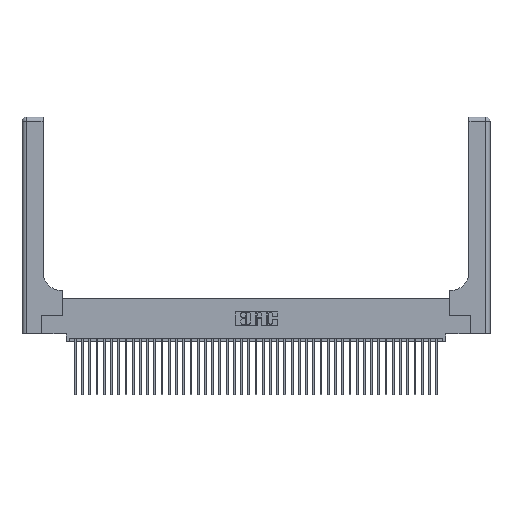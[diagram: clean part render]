
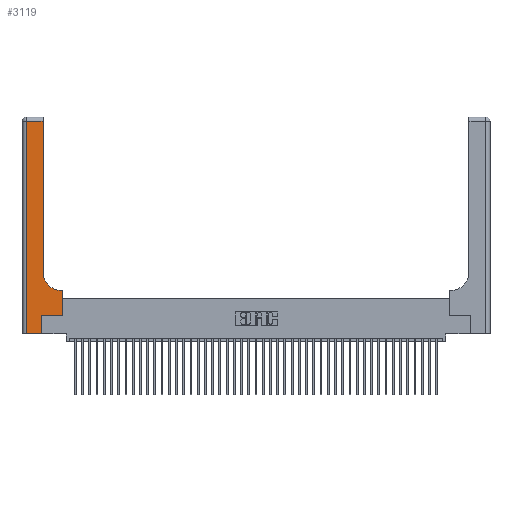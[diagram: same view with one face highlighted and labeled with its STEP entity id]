
A CAD part, top view. The second image highlights one B-rep face of the part: STEP entity #3119.
In plain terms, the highlighted planar face has unit normal (0, 0, 1).
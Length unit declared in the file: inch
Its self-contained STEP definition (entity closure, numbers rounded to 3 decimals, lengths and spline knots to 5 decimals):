
#1392 = CARTESIAN_POINT ( 'NONE',  ( 0.5415, 0.85, 0.37 ) ) ;
#1647 = DIRECTION ( 'NONE',  ( 0., 1., 0. ) ) ;
#1815 = CARTESIAN_POINT ( 'NONE',  ( 0.2915, 0.85, 0.37 ) ) ;
#2282 = EDGE_CURVE ( 'NONE', #7148, #27788, #36625, .T. ) ;
#2866 = VERTEX_POINT ( 'NONE', #33381 ) ;
#3119 = ADVANCED_FACE ( 'NONE', ( #38678 ), #14291, .F. ) ;
#3980 = DIRECTION ( 'NONE',  ( 0., 0., -1. ) ) ;
#4210 = CARTESIAN_POINT ( 'NONE',  ( 0.2915, 3., 0.37 ) ) ;
#4377 = CARTESIAN_POINT ( 'NONE',  ( 0.269, 0.25, 0.37 ) ) ;
#4675 = CARTESIAN_POINT ( 'NONE',  ( 0.06, 3., 0.37 ) ) ;
#4751 = VERTEX_POINT ( 'NONE', #36225 ) ;
#4891 = DIRECTION ( 'NONE',  ( 1., 0., 0. ) ) ;
#5026 = EDGE_LOOP ( 'NONE', ( #21530, #34138, #6974, #40006, #12952, #43656, #7484, #37822, #17677 ) ) ;
#5408 = CARTESIAN_POINT ( 'NONE',  ( 0., 0., 0.37 ) ) ;
#5466 = CARTESIAN_POINT ( 'NONE',  ( 0., 2.94, 0.37 ) ) ;
#6088 = VECTOR ( 'NONE', #18332, 39.37008 ) ;
#6974 = ORIENTED_EDGE ( 'NONE', *, *, #28302, .T. ) ;
#7148 = VERTEX_POINT ( 'NONE', #40310 ) ;
#7484 = ORIENTED_EDGE ( 'NONE', *, *, #22381, .T. ) ;
#9684 = VERTEX_POINT ( 'NONE', #41840 ) ;
#10985 = EDGE_CURVE ( 'NONE', #23581, #28740, #34920, .T. ) ;
#12034 = LINE ( 'NONE', #5408, #29040 ) ;
#12522 = EDGE_CURVE ( 'NONE', #38321, #9684, #15278, .T. ) ;
#12952 = ORIENTED_EDGE ( 'NONE', *, *, #2282, .T. ) ;
#13317 = DIRECTION ( 'NONE',  ( 0., 1., 0. ) ) ;
#13901 = CARTESIAN_POINT ( 'NONE',  ( 0.2915, 2.94, 0.37 ) ) ;
#14291 = PLANE ( 'NONE',  #16035 ) ;
#14669 = DIRECTION ( 'NONE',  ( 1., 0., 0. ) ) ;
#15278 = LINE ( 'NONE', #42009, #6088 ) ;
#15535 = EDGE_CURVE ( 'NONE', #9684, #23581, #39375, .T. ) ;
#16035 = AXIS2_PLACEMENT_3D ( 'NONE', #41349, #3980, #27906 ) ;
#17169 = VECTOR ( 'NONE', #28577, 39.37008 ) ;
#17677 = ORIENTED_EDGE ( 'NONE', *, *, #15535, .T. ) ;
#17799 = EDGE_CURVE ( 'NONE', #28740, #27933, #38593, .T. ) ;
#17800 = LINE ( 'NONE', #4377, #35816 ) ;
#17976 = VECTOR ( 'NONE', #24683, 39.37008 ) ;
#18332 = DIRECTION ( 'NONE',  ( -1., 0., 0. ) ) ;
#18610 = VECTOR ( 'NONE', #13317, 39.37008 ) ;
#19510 = VECTOR ( 'NONE', #29352, 39.37008 ) ;
#21420 = CARTESIAN_POINT ( 'NONE',  ( 0.5585, 0.6, 0.37 ) ) ;
#21530 = ORIENTED_EDGE ( 'NONE', *, *, #10985, .T. ) ;
#22381 = EDGE_CURVE ( 'NONE', #4751, #38321, #26546, .T. ) ;
#23581 = VERTEX_POINT ( 'NONE', #1815 ) ;
#24683 = DIRECTION ( 'NONE',  ( 0., 1., 0. ) ) ;
#25368 = DIRECTION ( 'NONE',  ( 0., 0., -1. ) ) ;
#25462 = CARTESIAN_POINT ( 'NONE',  ( 0.5585, 0.25, 0.37 ) ) ;
#26464 = EDGE_CURVE ( 'NONE', #27788, #4751, #17800, .T. ) ;
#26546 = LINE ( 'NONE', #25462, #34482 ) ;
#26779 = CARTESIAN_POINT ( 'NONE',  ( 0.269, 0., 0.37 ) ) ;
#27788 = VERTEX_POINT ( 'NONE', #29080 ) ;
#27906 = DIRECTION ( 'NONE',  ( -1., 0., 0. ) ) ;
#27933 = VERTEX_POINT ( 'NONE', #29805 ) ;
#28302 = EDGE_CURVE ( 'NONE', #27933, #2866, #36246, .T. ) ;
#28577 = DIRECTION ( 'NONE',  ( 0., -1., 0. ) ) ;
#28740 = VERTEX_POINT ( 'NONE', #13901 ) ;
#29040 = VECTOR ( 'NONE', #42901, 39.37008 ) ;
#29080 = CARTESIAN_POINT ( 'NONE',  ( 0.269, 0.25, 0.37 ) ) ;
#29352 = DIRECTION ( 'NONE',  ( -1., 0., 0. ) ) ;
#29660 = AXIS2_PLACEMENT_3D ( 'NONE', #1392, #25368, #4891 ) ;
#29805 = CARTESIAN_POINT ( 'NONE',  ( 0.06, 2.94, 0.37 ) ) ;
#33381 = CARTESIAN_POINT ( 'NONE',  ( 0.06, 0., 0.37 ) ) ;
#34138 = ORIENTED_EDGE ( 'NONE', *, *, #17799, .T. ) ;
#34482 = VECTOR ( 'NONE', #1647, 39.37008 ) ;
#34920 = LINE ( 'NONE', #4210, #17976 ) ;
#35816 = VECTOR ( 'NONE', #14669, 39.37008 ) ;
#36225 = CARTESIAN_POINT ( 'NONE',  ( 0.5585, 0.25, 0.37 ) ) ;
#36246 = LINE ( 'NONE', #4675, #17169 ) ;
#36625 = LINE ( 'NONE', #26779, #18610 ) ;
#37822 = ORIENTED_EDGE ( 'NONE', *, *, #12522, .T. ) ;
#38040 = EDGE_CURVE ( 'NONE', #2866, #7148, #12034, .T. ) ;
#38321 = VERTEX_POINT ( 'NONE', #21420 ) ;
#38593 = LINE ( 'NONE', #5466, #19510 ) ;
#38678 = FACE_OUTER_BOUND ( 'NONE', #5026, .T. ) ;
#39375 = CIRCLE ( 'NONE', #29660, 0.25 ) ;
#40006 = ORIENTED_EDGE ( 'NONE', *, *, #38040, .T. ) ;
#40310 = CARTESIAN_POINT ( 'NONE',  ( 0.269, 0., 0.37 ) ) ;
#41349 = CARTESIAN_POINT ( 'NONE',  ( 0., 3., 0.37 ) ) ;
#41840 = CARTESIAN_POINT ( 'NONE',  ( 0.5415, 0.6, 0.37 ) ) ;
#42009 = CARTESIAN_POINT ( 'NONE',  ( 0.2915, 0.6, 0.37 ) ) ;
#42901 = DIRECTION ( 'NONE',  ( 1., 0., 0. ) ) ;
#43656 = ORIENTED_EDGE ( 'NONE', *, *, #26464, .T. ) ;
